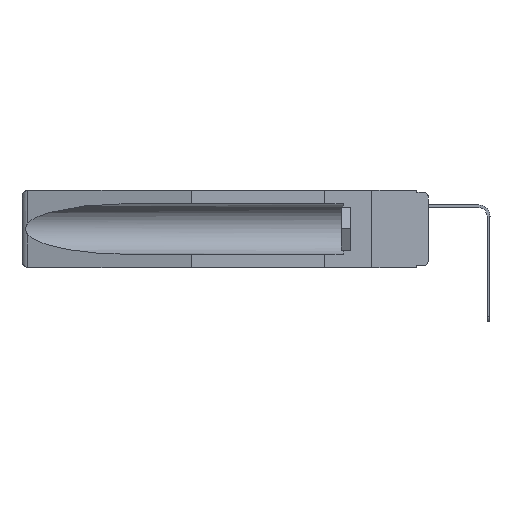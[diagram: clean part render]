
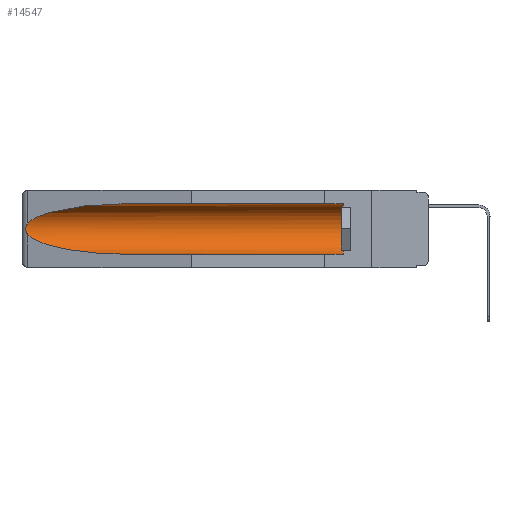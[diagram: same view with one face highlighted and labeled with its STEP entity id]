
A CAD part, left-side view. The second image highlights one B-rep face of the part: STEP entity #14547.
In plain terms, the highlighted cylindrical face has radius 2.857 mm (diameter 5.715 mm), a partial arc.
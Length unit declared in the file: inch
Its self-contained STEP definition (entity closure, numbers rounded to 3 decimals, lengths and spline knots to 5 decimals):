
#856 = CARTESIAN_POINT ( 'NONE',  ( 0.26654, 1.53092, -0.15636 ) ) ;
#976 = CARTESIAN_POINT ( 'NONE',  ( 0.155, 1.07973, -0.059 ) ) ;
#1095 = ORIENTED_EDGE ( 'NONE', *, *, #15572, .T. ) ;
#1151 = CYLINDRICAL_SURFACE ( 'NONE', #7288, 0.1125 ) ;
#1425 = VERTEX_POINT ( 'NONE', #976 ) ;
#1574 = AXIS2_PLACEMENT_3D ( 'NONE', #5370, #11281, #2636 ) ;
#2100 = LINE ( 'NONE', #4204, #17906 ) ;
#2392 = CARTESIAN_POINT ( 'NONE',  ( 0.21114, 1.30732, -0.284 ) ) ;
#2511 = CARTESIAN_POINT ( 'NONE',  ( 0.155, -0.30754, -0.1715 ) ) ;
#2636 = DIRECTION ( 'NONE',  ( 0., 0., 1. ) ) ;
#2748 = ORIENTED_EDGE ( 'NONE', *, *, #14468, .T. ) ;
#2862 = ORIENTED_EDGE ( 'NONE', *, *, #10012, .F. ) ;
#3741 = CARTESIAN_POINT ( 'NONE',  ( 0.155, 1.07973, -0.284 ) ) ;
#4034 = EDGE_LOOP ( 'NONE', ( #5264, #13784, #5242, #2862, #2748, #1095 ) ) ;
#4204 = CARTESIAN_POINT ( 'NONE',  ( 0.155, -0.30754, -0.284 ) ) ;
#4335 = CARTESIAN_POINT ( 'NONE',  ( 0.155, 0.126, -0.284 ) ) ;
#4519 = CARTESIAN_POINT ( 'NONE',  ( 0.26537, 1.52718, -0.19328 ) ) ;
#4900 = CARTESIAN_POINT ( 'NONE',  ( 0.155, -0.30754, -0.059 ) ) ;
#5242 = ORIENTED_EDGE ( 'NONE', *, *, #13865, .T. ) ;
#5264 = ORIENTED_EDGE ( 'NONE', *, *, #15167, .T. ) ;
#5292 = CARTESIAN_POINT ( 'NONE',  ( 0.26537, 1.52718, -0.14972 ) ) ;
#5370 = CARTESIAN_POINT ( 'NONE',  ( 0.155, 0.126, -0.1715 ) ) ;
#5538 = CARTESIAN_POINT ( 'NONE',  ( 0.21114, 1.30732, -0.059 ) ) ;
#6437 = CARTESIAN_POINT ( 'NONE',  ( 0.26655, 1.53094, -0.18657 ) ) ;
#6576 = FACE_OUTER_BOUND ( 'NONE', #4034, .T. ) ;
#6633 = CARTESIAN_POINT ( 'NONE',  ( 0.26537, 1.52718, -0.19328 ) ) ;
#6666 = CARTESIAN_POINT ( 'NONE',  ( 0.155, 0.126, -0.059 ) ) ;
#6995 =( BOUNDED_CURVE ( )  B_SPLINE_CURVE ( 3, ( #17000, #5538, #8344, #18471 ),
 .UNSPECIFIED., .F., .F. ) 
 B_SPLINE_CURVE_WITH_KNOTS ( ( 4, 4 ),
 ( 4.71239, 6.08839 ),
 .UNSPECIFIED. ) 
 CURVE ( )  GEOMETRIC_REPRESENTATION_ITEM ( )  RATIONAL_B_SPLINE_CURVE ( ( 1., 0.848, 0.848, 1. ) ) 
 REPRESENTATION_ITEM ( '' )  );
#6999 = LINE ( 'NONE', #4900, #11489 ) ;
#7288 = AXIS2_PLACEMENT_3D ( 'NONE', #2511, #15467, #15523 ) ;
#7816 = CARTESIAN_POINT ( 'NONE',  ( 0.26597, 1.52961, -0.15275 ) ) ;
#7872 = VERTEX_POINT ( 'NONE', #5292 ) ;
#8060 = CARTESIAN_POINT ( 'NONE',  ( 0.2675, 1.53308, -0.16763 ) ) ;
#8065 = CARTESIAN_POINT ( 'NONE',  ( 0.25451, 1.48313, -0.24835 ) ) ;
#8344 = CARTESIAN_POINT ( 'NONE',  ( 0.25451, 1.48313, -0.09465 ) ) ;
#8364 = VERTEX_POINT ( 'NONE', #6666 ) ;
#8722 = EDGE_CURVE ( 'NONE', #7872, #12991, #10331, .T. ) ;
#9282 = DIRECTION ( 'NONE',  ( 0., 1., 0. ) ) ;
#9385 = CARTESIAN_POINT ( 'NONE',  ( 0.26537, 1.52718, -0.19328 ) ) ;
#10012 = EDGE_CURVE ( 'NONE', #12902, #15281, #2100, .T. ) ;
#10331 = B_SPLINE_CURVE_WITH_KNOTS ( 'NONE', 3,
 ( #16708, #7816, #856, #10974, #8060, #15273, #12409, #6437, #17910, #9385 ),
 .UNSPECIFIED., .F., .F.,
 ( 4, 2, 2, 2, 4 ),
 ( 0., 0.00029, 0.00058, 0.00087, 0.00117 ),
 .UNSPECIFIED. ) ;
#10813 =( BOUNDED_CURVE ( )  B_SPLINE_CURVE ( 3, ( #6633, #8065, #2392, #3741 ),
 .UNSPECIFIED., .F., .F. ) 
 B_SPLINE_CURVE_WITH_KNOTS ( ( 4, 4 ),
 ( 0.1948, 1.5708 ),
 .UNSPECIFIED. ) 
 CURVE ( )  GEOMETRIC_REPRESENTATION_ITEM ( )  RATIONAL_B_SPLINE_CURVE ( ( 1., 0.848, 0.848, 1. ) ) 
 REPRESENTATION_ITEM ( '' )  );
#10974 = CARTESIAN_POINT ( 'NONE',  ( 0.2673, 1.5327, -0.16383 ) ) ;
#11281 = DIRECTION ( 'NONE',  ( 0., -1., 0. ) ) ;
#11489 = VECTOR ( 'NONE', #9282, 39.37008 ) ;
#12409 = CARTESIAN_POINT ( 'NONE',  ( 0.2673, 1.53269, -0.17917 ) ) ;
#12658 = CIRCLE ( 'NONE', #1574, 0.1125 ) ;
#12902 = VERTEX_POINT ( 'NONE', #4335 ) ;
#12991 = VERTEX_POINT ( 'NONE', #4519 ) ;
#13121 = CARTESIAN_POINT ( 'NONE',  ( 0.155, 1.07973, -0.284 ) ) ;
#13784 = ORIENTED_EDGE ( 'NONE', *, *, #8722, .T. ) ;
#13865 = EDGE_CURVE ( 'NONE', #12991, #15281, #10813, .T. ) ;
#14281 = DIRECTION ( 'NONE',  ( 0., 1., 0. ) ) ;
#14468 = EDGE_CURVE ( 'NONE', #12902, #8364, #12658, .T. ) ;
#14547 = ADVANCED_FACE ( 'NONE', ( #6576 ), #1151, .F. ) ;
#15167 = EDGE_CURVE ( 'NONE', #1425, #7872, #6995, .T. ) ;
#15273 = CARTESIAN_POINT ( 'NONE',  ( 0.2675, 1.53308, -0.17534 ) ) ;
#15281 = VERTEX_POINT ( 'NONE', #13121 ) ;
#15467 = DIRECTION ( 'NONE',  ( 0., 1., 0. ) ) ;
#15523 = DIRECTION ( 'NONE',  ( 0., 0., 1. ) ) ;
#15572 = EDGE_CURVE ( 'NONE', #8364, #1425, #6999, .T. ) ;
#16708 = CARTESIAN_POINT ( 'NONE',  ( 0.26537, 1.52718, -0.14972 ) ) ;
#17000 = CARTESIAN_POINT ( 'NONE',  ( 0.155, 1.07973, -0.059 ) ) ;
#17906 = VECTOR ( 'NONE', #14281, 39.37008 ) ;
#17910 = CARTESIAN_POINT ( 'NONE',  ( 0.26597, 1.5296, -0.19026 ) ) ;
#18471 = CARTESIAN_POINT ( 'NONE',  ( 0.26537, 1.52718, -0.14972 ) ) ;
